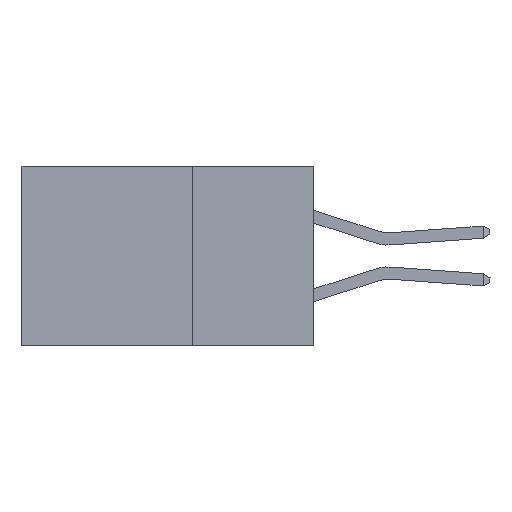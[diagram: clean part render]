
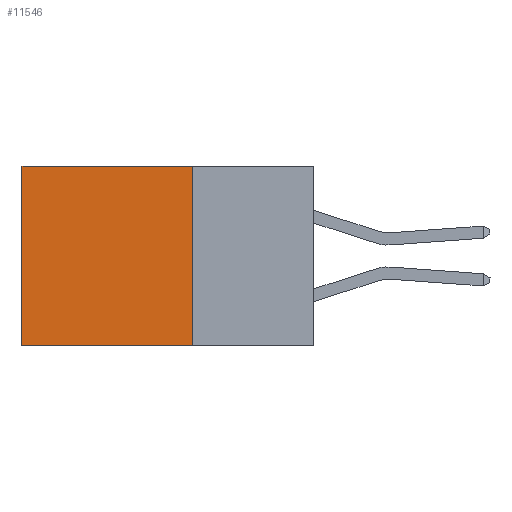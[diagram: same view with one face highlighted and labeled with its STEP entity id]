
A CAD part, left-side view. The second image highlights one B-rep face of the part: STEP entity #11546.
In plain terms, the highlighted planar face has unit normal (-1, 0, 0).
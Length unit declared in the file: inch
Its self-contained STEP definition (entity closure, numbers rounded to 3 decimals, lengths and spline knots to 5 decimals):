
#89 = VECTOR ( 'NONE', #5462, 39.37008 ) ;
#810 = DIRECTION ( 'NONE',  ( 0., 1., 0. ) ) ;
#1245 = EDGE_CURVE ( 'NONE', #5144, #1253, #9752, .T. ) ;
#1253 = VERTEX_POINT ( 'NONE', #2482 ) ;
#1858 = ORIENTED_EDGE ( 'NONE', *, *, #9140, .T. ) ;
#2149 = VERTEX_POINT ( 'NONE', #4089 ) ;
#2369 = FACE_OUTER_BOUND ( 'NONE', #14980, .T. ) ;
#2482 = CARTESIAN_POINT ( 'NONE',  ( 0.2875, 0.25, -0.37 ) ) ;
#2747 = ORIENTED_EDGE ( 'NONE', *, *, #14266, .F. ) ;
#3306 = CARTESIAN_POINT ( 'NONE',  ( 0.2875, 0.25, -0.37 ) ) ;
#3927 = LINE ( 'NONE', #3306, #12594 ) ;
#4089 = CARTESIAN_POINT ( 'NONE',  ( 0.2875, 0.6, -0.37 ) ) ;
#4094 = VECTOR ( 'NONE', #5092, 39.37008 ) ;
#4627 = CARTESIAN_POINT ( 'NONE',  ( 0.2875, 0.25, 0. ) ) ;
#5092 = DIRECTION ( 'NONE',  ( 0., 0., -1. ) ) ;
#5144 = VERTEX_POINT ( 'NONE', #11140 ) ;
#5462 = DIRECTION ( 'NONE',  ( 0., 0., -1. ) ) ;
#5763 = VECTOR ( 'NONE', #10945, 39.37008 ) ;
#5965 = ORIENTED_EDGE ( 'NONE', *, *, #8617, .T. ) ;
#8425 = CARTESIAN_POINT ( 'NONE',  ( 0.2875, 0.25, 0. ) ) ;
#8617 = EDGE_CURVE ( 'NONE', #5144, #15476, #11413, .T. ) ;
#9140 = EDGE_CURVE ( 'NONE', #15476, #2149, #14016, .T. ) ;
#9222 = AXIS2_PLACEMENT_3D ( 'NONE', #4627, #14817, #14773 ) ;
#9752 = LINE ( 'NONE', #14271, #4094 ) ;
#10945 = DIRECTION ( 'NONE',  ( 0., 1., 0. ) ) ;
#11140 = CARTESIAN_POINT ( 'NONE',  ( 0.2875, 0.25, 0. ) ) ;
#11413 = LINE ( 'NONE', #8425, #5763 ) ;
#11546 = ADVANCED_FACE ( 'NONE', ( #2369 ), #13546, .F. ) ;
#11983 = CARTESIAN_POINT ( 'NONE',  ( 0.2875, 0.6, 0. ) ) ;
#12594 = VECTOR ( 'NONE', #810, 39.37008 ) ;
#13352 = CARTESIAN_POINT ( 'NONE',  ( 0.2875, 0.6, 0. ) ) ;
#13546 = PLANE ( 'NONE',  #9222 ) ;
#14016 = LINE ( 'NONE', #11983, #89 ) ;
#14266 = EDGE_CURVE ( 'NONE', #1253, #2149, #3927, .T. ) ;
#14271 = CARTESIAN_POINT ( 'NONE',  ( 0.2875, 0.25, 0. ) ) ;
#14773 = DIRECTION ( 'NONE',  ( 0., 0., -1. ) ) ;
#14817 = DIRECTION ( 'NONE',  ( 1., 0., 0. ) ) ;
#14980 = EDGE_LOOP ( 'NONE', ( #1858, #2747, #15320, #5965 ) ) ;
#15320 = ORIENTED_EDGE ( 'NONE', *, *, #1245, .F. ) ;
#15476 = VERTEX_POINT ( 'NONE', #13352 ) ;
